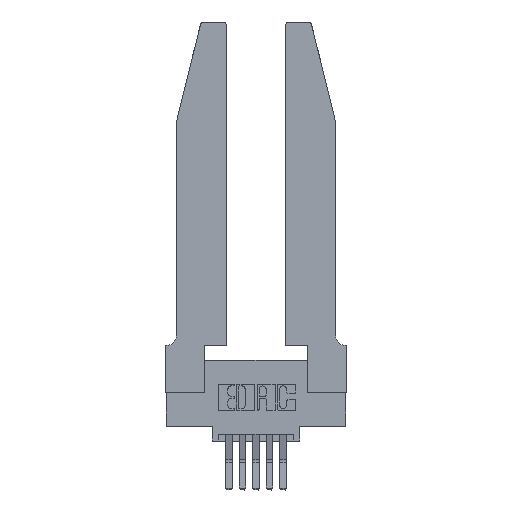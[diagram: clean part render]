
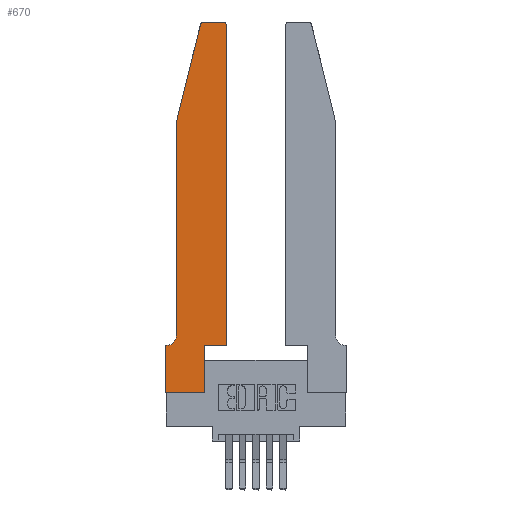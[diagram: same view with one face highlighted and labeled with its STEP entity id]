
A CAD part, top view. The second image highlights one B-rep face of the part: STEP entity #670.
In plain terms, the highlighted planar face has unit normal (0, 0, 1).
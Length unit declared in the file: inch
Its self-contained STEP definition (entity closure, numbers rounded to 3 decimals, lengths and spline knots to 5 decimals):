
#58 = LINE ( 'NONE', #7491, #13330 ) ;
#202 = LINE ( 'NONE', #7128, #2877 ) ;
#528 = EDGE_CURVE ( 'NONE', #12418, #7476, #10389, .T. ) ;
#670 = ADVANCED_FACE ( 'NONE', ( #10147 ), #3020, .T. ) ;
#679 = ORIENTED_EDGE ( 'NONE', *, *, #528, .T. ) ;
#783 = ORIENTED_EDGE ( 'NONE', *, *, #9003, .T. ) ;
#905 = DIRECTION ( 'NONE',  ( 1., 0., 0. ) ) ;
#1364 = VECTOR ( 'NONE', #12909, 39.37008 ) ;
#1509 = EDGE_CURVE ( 'NONE', #5073, #12428, #4691, .T. ) ;
#1725 = EDGE_CURVE ( 'NONE', #10563, #3103, #13856, .T. ) ;
#1966 = CARTESIAN_POINT ( 'NONE',  ( 0., 0.35, 0.37 ) ) ;
#2116 = DIRECTION ( 'NONE',  ( 0., -1., 0. ) ) ;
#2303 = VECTOR ( 'NONE', #11241, 39.37008 ) ;
#2794 = CARTESIAN_POINT ( 'NONE',  ( 0.0055, 0.42, 0.37 ) ) ;
#2850 = DIRECTION ( 'NONE',  ( 0., 0., 1. ) ) ;
#2877 = VECTOR ( 'NONE', #10279, 39.37008 ) ;
#3020 = PLANE ( 'NONE',  #4485 ) ;
#3103 = VERTEX_POINT ( 'NONE', #10845 ) ;
#3300 = CARTESIAN_POINT ( 'NONE',  ( 0.4505, 0.35, 0.37 ) ) ;
#3312 = CARTESIAN_POINT ( 'NONE',  ( 0.0755, 2., 0.37 ) ) ;
#3345 = DIRECTION ( 'NONE',  ( 1., 0., 0. ) ) ;
#3480 = DIRECTION ( 'NONE',  ( 0., 1., 0. ) ) ;
#3713 = CARTESIAN_POINT ( 'NONE',  ( 0.2865, 0.35, 0.37 ) ) ;
#3728 = VERTEX_POINT ( 'NONE', #5509 ) ;
#3909 = DIRECTION ( 'NONE',  ( -1., 0., 0. ) ) ;
#4013 = EDGE_CURVE ( 'NONE', #3728, #5073, #12688, .T. ) ;
#4093 = CARTESIAN_POINT ( 'NONE',  ( 0.25487, 2.72718, 0.37 ) ) ;
#4442 = DIRECTION ( 'NONE',  ( -0.239, -0.971, 0. ) ) ;
#4485 = AXIS2_PLACEMENT_3D ( 'NONE', #7952, #5960, #6000 ) ;
#4665 = VECTOR ( 'NONE', #4871, 39.37008 ) ;
#4691 = LINE ( 'NONE', #10838, #12742 ) ;
#4701 = EDGE_CURVE ( 'NONE', #8526, #8810, #202, .T. ) ;
#4792 = VECTOR ( 'NONE', #4442, 39.37008 ) ;
#4871 = DIRECTION ( 'NONE',  ( 1., 0., 0. ) ) ;
#4881 = AXIS2_PLACEMENT_3D ( 'NONE', #2794, #10252, #3909 ) ;
#5073 = VERTEX_POINT ( 'NONE', #13138 ) ;
#5131 = ORIENTED_EDGE ( 'NONE', *, *, #4013, .T. ) ;
#5241 = ORIENTED_EDGE ( 'NONE', *, *, #13257, .T. ) ;
#5411 = AXIS2_PLACEMENT_3D ( 'NONE', #13674, #7450, #905 ) ;
#5509 = CARTESIAN_POINT ( 'NONE',  ( 0.0755, 0.42, 0.37 ) ) ;
#5662 = ORIENTED_EDGE ( 'NONE', *, *, #1725, .T. ) ;
#5793 = ORIENTED_EDGE ( 'NONE', *, *, #10617, .T. ) ;
#5832 = EDGE_CURVE ( 'NONE', #8810, #10563, #10344, .T. ) ;
#5960 = DIRECTION ( 'NONE',  ( 0., 0., 1. ) ) ;
#6000 = DIRECTION ( 'NONE',  ( 1., 0., 0. ) ) ;
#7114 = CARTESIAN_POINT ( 'NONE',  ( 0.4505, 0.35, 0.37 ) ) ;
#7128 = CARTESIAN_POINT ( 'NONE',  ( 0.4505, 0.35, 0.37 ) ) ;
#7134 = LINE ( 'NONE', #8739, #1364 ) ;
#7450 = DIRECTION ( 'NONE',  ( 0., 0., 1. ) ) ;
#7476 = VERTEX_POINT ( 'NONE', #10410 ) ;
#7491 = CARTESIAN_POINT ( 'NONE',  ( 0.0755, 2., 0.37 ) ) ;
#7571 = CIRCLE ( 'NONE', #11424, 0.03 ) ;
#7952 = CARTESIAN_POINT ( 'NONE',  ( 0., 0.35, 0.37 ) ) ;
#7989 = ORIENTED_EDGE ( 'NONE', *, *, #1509, .T. ) ;
#8526 = VERTEX_POINT ( 'NONE', #7114 ) ;
#8634 = ORIENTED_EDGE ( 'NONE', *, *, #4701, .T. ) ;
#8739 = CARTESIAN_POINT ( 'NONE',  ( 0., 0., 0.37 ) ) ;
#8810 = VERTEX_POINT ( 'NONE', #13800 ) ;
#8869 = ORIENTED_EDGE ( 'NONE', *, *, #5832, .T. ) ;
#9003 = EDGE_CURVE ( 'NONE', #11391, #12418, #12410, .T. ) ;
#9089 = DIRECTION ( 'NONE',  ( -1., 0., 0. ) ) ;
#9160 = ORIENTED_EDGE ( 'NONE', *, *, #9717, .T. ) ;
#9261 = CARTESIAN_POINT ( 'NONE',  ( 0.284, 2.72, 0.37 ) ) ;
#9711 = CARTESIAN_POINT ( 'NONE',  ( 0., 0., 0.37 ) ) ;
#9717 = EDGE_CURVE ( 'NONE', #7476, #8526, #13038, .T. ) ;
#10147 = FACE_OUTER_BOUND ( 'NONE', #11511, .T. ) ;
#10252 = DIRECTION ( 'NONE',  ( 0., 0., -1. ) ) ;
#10265 = VECTOR ( 'NONE', #3345, 39.37008 ) ;
#10279 = DIRECTION ( 'NONE',  ( 0., 1., 0. ) ) ;
#10301 = DIRECTION ( 'NONE',  ( 1., 0., 0. ) ) ;
#10344 = CIRCLE ( 'NONE', #5411, 0.03 ) ;
#10348 = CARTESIAN_POINT ( 'NONE',  ( 0.0755, 2., 0.37 ) ) ;
#10389 = LINE ( 'NONE', #3713, #10730 ) ;
#10407 = CARTESIAN_POINT ( 'NONE',  ( 0.4205, 2.75, 0.37 ) ) ;
#10410 = CARTESIAN_POINT ( 'NONE',  ( 0.2865, 0.35, 0.37 ) ) ;
#10447 = CARTESIAN_POINT ( 'NONE',  ( 0.2865, 0., 0.37 ) ) ;
#10469 = CARTESIAN_POINT ( 'NONE',  ( 0.2605, 2.75, 0.37 ) ) ;
#10563 = VERTEX_POINT ( 'NONE', #10407 ) ;
#10617 = EDGE_CURVE ( 'NONE', #13309, #3728, #58, .T. ) ;
#10730 = VECTOR ( 'NONE', #3480, 39.37008 ) ;
#10758 = EDGE_CURVE ( 'NONE', #12428, #11391, #7134, .T. ) ;
#10838 = CARTESIAN_POINT ( 'NONE',  ( 0.0755, 0.35, 0.37 ) ) ;
#10845 = CARTESIAN_POINT ( 'NONE',  ( 0.284, 2.75, 0.37 ) ) ;
#11115 = ORIENTED_EDGE ( 'NONE', *, *, #10758, .T. ) ;
#11199 = CARTESIAN_POINT ( 'NONE',  ( 0., 0., 0.37 ) ) ;
#11241 = DIRECTION ( 'NONE',  ( -1., 0., 0. ) ) ;
#11391 = VERTEX_POINT ( 'NONE', #9711 ) ;
#11400 = EDGE_CURVE ( 'NONE', #11831, #13309, #13152, .T. ) ;
#11424 = AXIS2_PLACEMENT_3D ( 'NONE', #9261, #2850, #10301 ) ;
#11511 = EDGE_LOOP ( 'NONE', ( #5662, #5241, #12194, #5793, #5131, #7989, #11115, #783, #679, #9160, #8634, #8869 ) ) ;
#11831 = VERTEX_POINT ( 'NONE', #4093 ) ;
#12194 = ORIENTED_EDGE ( 'NONE', *, *, #11400, .T. ) ;
#12410 = LINE ( 'NONE', #11199, #4665 ) ;
#12418 = VERTEX_POINT ( 'NONE', #10447 ) ;
#12428 = VERTEX_POINT ( 'NONE', #1966 ) ;
#12688 = CIRCLE ( 'NONE', #4881, 0.07 ) ;
#12742 = VECTOR ( 'NONE', #9089, 39.37008 ) ;
#12909 = DIRECTION ( 'NONE',  ( 0., -1., 0. ) ) ;
#13038 = LINE ( 'NONE', #3300, #10265 ) ;
#13138 = CARTESIAN_POINT ( 'NONE',  ( 0.0055, 0.35, 0.37 ) ) ;
#13152 = LINE ( 'NONE', #3312, #4792 ) ;
#13257 = EDGE_CURVE ( 'NONE', #3103, #11831, #7571, .T. ) ;
#13309 = VERTEX_POINT ( 'NONE', #10348 ) ;
#13330 = VECTOR ( 'NONE', #2116, 39.37008 ) ;
#13674 = CARTESIAN_POINT ( 'NONE',  ( 0.4205, 2.72, 0.37 ) ) ;
#13800 = CARTESIAN_POINT ( 'NONE',  ( 0.4505, 2.72, 0.37 ) ) ;
#13856 = LINE ( 'NONE', #10469, #2303 ) ;
